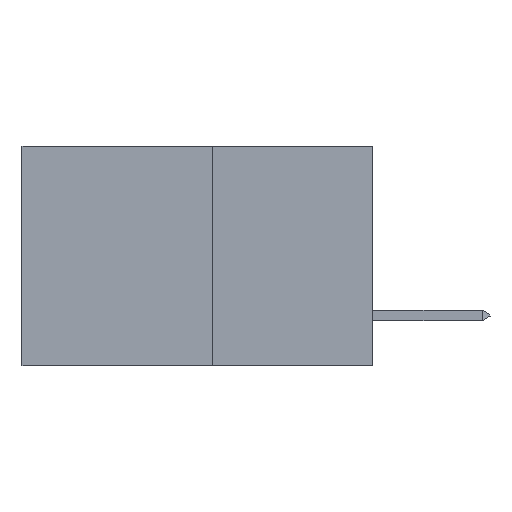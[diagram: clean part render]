
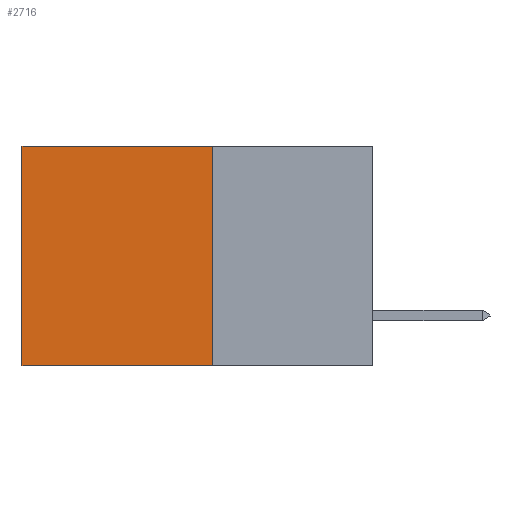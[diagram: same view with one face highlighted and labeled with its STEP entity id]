
A CAD part, left-side view. The second image highlights one B-rep face of the part: STEP entity #2716.
In plain terms, the highlighted planar face has unit normal (-1, 0, 0).
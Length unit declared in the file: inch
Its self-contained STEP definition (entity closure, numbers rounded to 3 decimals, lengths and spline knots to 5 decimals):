
#691 = VECTOR ( 'NONE', #9911, 39.37008 ) ;
#701 = DIRECTION ( 'NONE',  ( 0., 1., 0. ) ) ;
#1011 = LINE ( 'NONE', #12003, #691 ) ;
#1124 = VERTEX_POINT ( 'NONE', #7049 ) ;
#1409 = ORIENTED_EDGE ( 'NONE', *, *, #3601, .T. ) ;
#1589 = DIRECTION ( 'NONE',  ( 0., 0., -1. ) ) ;
#1668 = VERTEX_POINT ( 'NONE', #7990 ) ;
#2213 = AXIS2_PLACEMENT_3D ( 'NONE', #3282, #3181, #2995 ) ;
#2417 = EDGE_LOOP ( 'NONE', ( #4023, #7091, #7368, #1409 ) ) ;
#2476 = VECTOR ( 'NONE', #701, 39.37008 ) ;
#2580 = CARTESIAN_POINT ( 'NONE',  ( 0.277, 0.27, 0. ) ) ;
#2716 = ADVANCED_FACE ( 'NONE', ( #12104 ), #3345, .F. ) ;
#2995 = DIRECTION ( 'NONE',  ( 0., 0., -1. ) ) ;
#3181 = DIRECTION ( 'NONE',  ( 1., 0., 0. ) ) ;
#3282 = CARTESIAN_POINT ( 'NONE',  ( 0.277, 0.27, -0.37 ) ) ;
#3345 = PLANE ( 'NONE',  #2213 ) ;
#3601 = EDGE_CURVE ( 'NONE', #1668, #5559, #7157, .T. ) ;
#3656 = DIRECTION ( 'NONE',  ( 0., 1., 0. ) ) ;
#3874 = CARTESIAN_POINT ( 'NONE',  ( 0.277, 0.27, -0.37 ) ) ;
#4023 = ORIENTED_EDGE ( 'NONE', *, *, #7744, .T. ) ;
#5559 = VERTEX_POINT ( 'NONE', #13472 ) ;
#5916 = VERTEX_POINT ( 'NONE', #13036 ) ;
#5925 = VECTOR ( 'NONE', #1589, 39.37008 ) ;
#6809 = VECTOR ( 'NONE', #3656, 39.37008 ) ;
#7049 = CARTESIAN_POINT ( 'NONE',  ( 0.277, 0.27, -0.37 ) ) ;
#7091 = ORIENTED_EDGE ( 'NONE', *, *, #12856, .F. ) ;
#7157 = LINE ( 'NONE', #2580, #6809 ) ;
#7368 = ORIENTED_EDGE ( 'NONE', *, *, #7480, .F. ) ;
#7480 = EDGE_CURVE ( 'NONE', #1668, #1124, #1011, .T. ) ;
#7744 = EDGE_CURVE ( 'NONE', #5559, #5916, #9470, .T. ) ;
#7990 = CARTESIAN_POINT ( 'NONE',  ( 0.277, 0.27, 0. ) ) ;
#8965 = LINE ( 'NONE', #3874, #2476 ) ;
#9182 = CARTESIAN_POINT ( 'NONE',  ( 0.277, 0.59, -0.37 ) ) ;
#9470 = LINE ( 'NONE', #9182, #5925 ) ;
#9911 = DIRECTION ( 'NONE',  ( 0., 0., -1. ) ) ;
#12003 = CARTESIAN_POINT ( 'NONE',  ( 0.277, 0.27, -0.37 ) ) ;
#12104 = FACE_OUTER_BOUND ( 'NONE', #2417, .T. ) ;
#12856 = EDGE_CURVE ( 'NONE', #1124, #5916, #8965, .T. ) ;
#13036 = CARTESIAN_POINT ( 'NONE',  ( 0.277, 0.59, -0.37 ) ) ;
#13472 = CARTESIAN_POINT ( 'NONE',  ( 0.277, 0.59, 0. ) ) ;
